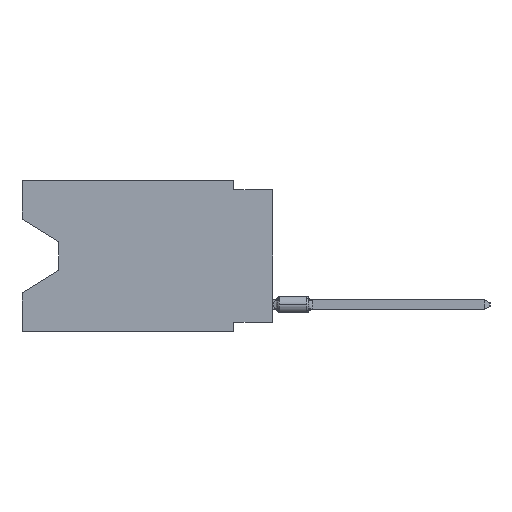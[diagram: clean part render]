
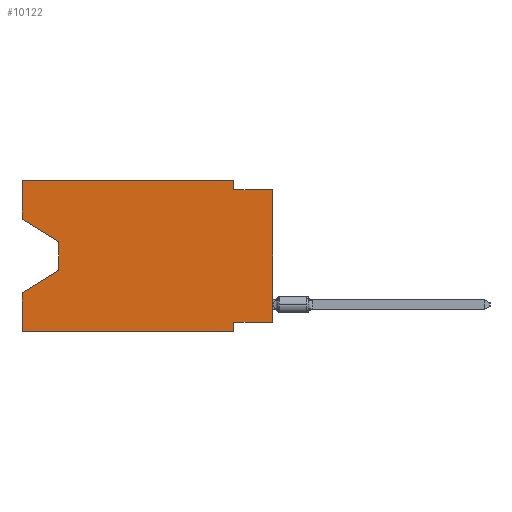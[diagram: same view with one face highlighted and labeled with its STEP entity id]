
A CAD part, left-side view. The second image highlights one B-rep face of the part: STEP entity #10122.
In plain terms, the highlighted planar face has unit normal (-1, 0, 0).
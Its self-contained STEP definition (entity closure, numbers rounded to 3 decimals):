
#400 = VERTEX_POINT ( 'NONE', #14045 ) ;
#3399 = DIRECTION ( 'NONE',  ( 0., 0., -1. ) ) ;
#4704 = VECTOR ( 'NONE', #36595, 1000. ) ;
#5859 = EDGE_CURVE ( 'NONE', #40475, #50788, #24075, .T. ) ;
#5905 = DIRECTION ( 'NONE',  ( 0., 0., -1. ) ) ;
#6091 = ORIENTED_EDGE ( 'NONE', *, *, #43152, .T. ) ;
#6932 = CARTESIAN_POINT ( 'NONE',  ( 0., 0., -0.635 ) ) ;
#7074 = LINE ( 'NONE', #32542, #7973 ) ;
#7436 = CARTESIAN_POINT ( 'NONE',  ( 0., 13.97, -4.013 ) ) ;
#7729 = AXIS2_PLACEMENT_3D ( 'NONE', #40545, #10196, #5905 ) ;
#7817 = VERTEX_POINT ( 'NONE', #35126 ) ;
#7973 = VECTOR ( 'NONE', #23386, 1000. ) ;
#8211 = CARTESIAN_POINT ( 'NONE',  ( 0., 0., 0. ) ) ;
#8278 = EDGE_CURVE ( 'NONE', #50788, #34405, #36304, .T. ) ;
#8530 = CARTESIAN_POINT ( 'NONE',  ( 0., 0., -0.635 ) ) ;
#9319 = LINE ( 'NONE', #8211, #20538 ) ;
#10122 = ADVANCED_FACE ( 'NONE', ( #15348 ), #49443, .F. ) ;
#10196 = DIRECTION ( 'NONE',  ( 1., 0., 0. ) ) ;
#10280 = VECTOR ( 'NONE', #56206, 1000. ) ;
#10460 = VECTOR ( 'NONE', #51971, 1000. ) ;
#11009 = VERTEX_POINT ( 'NONE', #47653 ) ;
#11381 = EDGE_CURVE ( 'NONE', #46162, #41589, #15224, .T. ) ;
#12138 = CARTESIAN_POINT ( 'NONE',  ( 0., 2.54, -9.906 ) ) ;
#14045 = CARTESIAN_POINT ( 'NONE',  ( 0., 13.97, -4.013 ) ) ;
#15224 = LINE ( 'NONE', #54750, #22515 ) ;
#15348 = FACE_OUTER_BOUND ( 'NONE', #44516, .T. ) ;
#16405 = CARTESIAN_POINT ( 'NONE',  ( 0., 16.383, -2.546 ) ) ;
#17404 = CARTESIAN_POINT ( 'NONE',  ( 0., 2.54, -9.271 ) ) ;
#17541 = EDGE_CURVE ( 'NONE', #19924, #7817, #37751, .T. ) ;
#19832 = EDGE_CURVE ( 'NONE', #43536, #400, #47904, .T. ) ;
#19924 = VERTEX_POINT ( 'NONE', #42746 ) ;
#20105 = ORIENTED_EDGE ( 'NONE', *, *, #53834, .F. ) ;
#20538 = VECTOR ( 'NONE', #43702, 1000. ) ;
#20759 = CARTESIAN_POINT ( 'NONE',  ( 0., 16.383, -9.906 ) ) ;
#21220 = LINE ( 'NONE', #56159, #45879 ) ;
#22515 = VECTOR ( 'NONE', #50184, 1000. ) ;
#22805 = CARTESIAN_POINT ( 'NONE',  ( 0., 16.383, 0. ) ) ;
#23386 = DIRECTION ( 'NONE',  ( 0., -1., 0. ) ) ;
#24075 = LINE ( 'NONE', #29791, #32880 ) ;
#24486 = VECTOR ( 'NONE', #31389, 1000. ) ;
#25438 = ORIENTED_EDGE ( 'NONE', *, *, #46659, .F. ) ;
#25614 = LINE ( 'NONE', #20759, #10460 ) ;
#25714 = CARTESIAN_POINT ( 'NONE',  ( 0., 2.54, 0. ) ) ;
#27155 = EDGE_CURVE ( 'NONE', #400, #46162, #51548, .T. ) ;
#29354 = VECTOR ( 'NONE', #3399, 1000. ) ;
#29791 = CARTESIAN_POINT ( 'NONE',  ( 0., 0., -9.271 ) ) ;
#30046 = DIRECTION ( 'NONE',  ( 0., 0., -1. ) ) ;
#31280 = ORIENTED_EDGE ( 'NONE', *, *, #56565, .F. ) ;
#31389 = DIRECTION ( 'NONE',  ( 0., 0., 1. ) ) ;
#32029 = VECTOR ( 'NONE', #30046, 1000. ) ;
#32542 = CARTESIAN_POINT ( 'NONE',  ( 0., 16.383, 0. ) ) ;
#32632 = EDGE_CURVE ( 'NONE', #40475, #50778, #9319, .T. ) ;
#32880 = VECTOR ( 'NONE', #37811, 1000. ) ;
#32978 = DIRECTION ( 'NONE',  ( 0., -1., 0. ) ) ;
#34405 = VERTEX_POINT ( 'NONE', #12138 ) ;
#35126 = CARTESIAN_POINT ( 'NONE',  ( 0., 2.54, -0.635 ) ) ;
#35247 = ORIENTED_EDGE ( 'NONE', *, *, #27155, .T. ) ;
#35898 = VECTOR ( 'NONE', #32978, 1000. ) ;
#35971 = CARTESIAN_POINT ( 'NONE',  ( 0., 16.383, 0. ) ) ;
#36304 = LINE ( 'NONE', #50368, #4704 ) ;
#36595 = DIRECTION ( 'NONE',  ( 0., 0., -1. ) ) ;
#37751 = LINE ( 'NONE', #25714, #29354 ) ;
#37811 = DIRECTION ( 'NONE',  ( 0., 1., 0. ) ) ;
#37876 = EDGE_CURVE ( 'NONE', #43536, #56582, #21220, .T. ) ;
#39309 = ORIENTED_EDGE ( 'NONE', *, *, #37876, .F. ) ;
#40432 = CARTESIAN_POINT ( 'NONE',  ( 0., 0., -9.271 ) ) ;
#40475 = VERTEX_POINT ( 'NONE', #40432 ) ;
#40545 = CARTESIAN_POINT ( 'NONE',  ( 0., 16.383, 0. ) ) ;
#41589 = VERTEX_POINT ( 'NONE', #54596 ) ;
#42746 = CARTESIAN_POINT ( 'NONE',  ( 0., 2.54, 0. ) ) ;
#42788 = ORIENTED_EDGE ( 'NONE', *, *, #32632, .T. ) ;
#43152 = EDGE_CURVE ( 'NONE', #11009, #34405, #25614, .T. ) ;
#43536 = VERTEX_POINT ( 'NONE', #50780 ) ;
#43702 = DIRECTION ( 'NONE',  ( 0., 0., 1. ) ) ;
#44516 = EDGE_LOOP ( 'NONE', ( #46813, #35247, #47351, #31280, #6091, #54698, #51310, #42788, #25438, #55844, #20105, #39309 ) ) ;
#45879 = VECTOR ( 'NONE', #47573, 1000. ) ;
#46162 = VERTEX_POINT ( 'NONE', #52597 ) ;
#46659 = EDGE_CURVE ( 'NONE', #7817, #50778, #49615, .T. ) ;
#46813 = ORIENTED_EDGE ( 'NONE', *, *, #19832, .T. ) ;
#47351 = ORIENTED_EDGE ( 'NONE', *, *, #11381, .T. ) ;
#47573 = DIRECTION ( 'NONE',  ( 0., 0., 1. ) ) ;
#47653 = CARTESIAN_POINT ( 'NONE',  ( 0., 16.383, -9.906 ) ) ;
#47904 = LINE ( 'NONE', #16405, #10280 ) ;
#49443 = PLANE ( 'NONE',  #7729 ) ;
#49446 = LINE ( 'NONE', #22805, #24486 ) ;
#49615 = LINE ( 'NONE', #6932, #35898 ) ;
#50184 = DIRECTION ( 'NONE',  ( 0., 0.855, -0.519 ) ) ;
#50368 = CARTESIAN_POINT ( 'NONE',  ( 0., 2.54, -9.906 ) ) ;
#50778 = VERTEX_POINT ( 'NONE', #8530 ) ;
#50780 = CARTESIAN_POINT ( 'NONE',  ( 0., 16.383, -2.546 ) ) ;
#50788 = VERTEX_POINT ( 'NONE', #17404 ) ;
#51310 = ORIENTED_EDGE ( 'NONE', *, *, #5859, .F. ) ;
#51548 = LINE ( 'NONE', #7436, #32029 ) ;
#51971 = DIRECTION ( 'NONE',  ( 0., -1., 0. ) ) ;
#52597 = CARTESIAN_POINT ( 'NONE',  ( 0., 13.97, -5.893 ) ) ;
#53834 = EDGE_CURVE ( 'NONE', #56582, #19924, #7074, .T. ) ;
#54596 = CARTESIAN_POINT ( 'NONE',  ( 0., 16.383, -7.36 ) ) ;
#54698 = ORIENTED_EDGE ( 'NONE', *, *, #8278, .F. ) ;
#54750 = CARTESIAN_POINT ( 'NONE',  ( 0., 13.97, -5.893 ) ) ;
#55844 = ORIENTED_EDGE ( 'NONE', *, *, #17541, .F. ) ;
#56159 = CARTESIAN_POINT ( 'NONE',  ( 0., 16.383, 0. ) ) ;
#56206 = DIRECTION ( 'NONE',  ( 0., -0.855, -0.519 ) ) ;
#56565 = EDGE_CURVE ( 'NONE', #11009, #41589, #49446, .T. ) ;
#56582 = VERTEX_POINT ( 'NONE', #35971 ) ;
